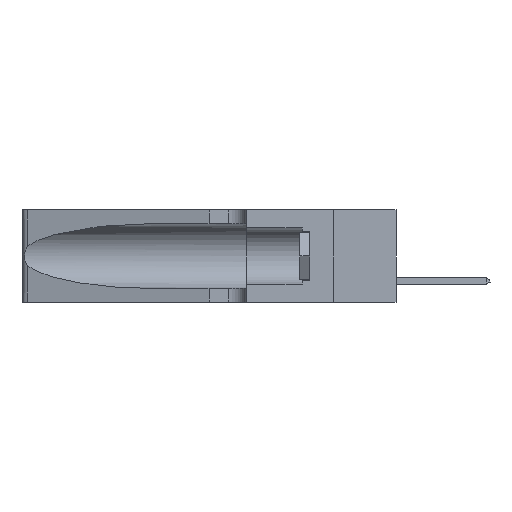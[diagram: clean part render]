
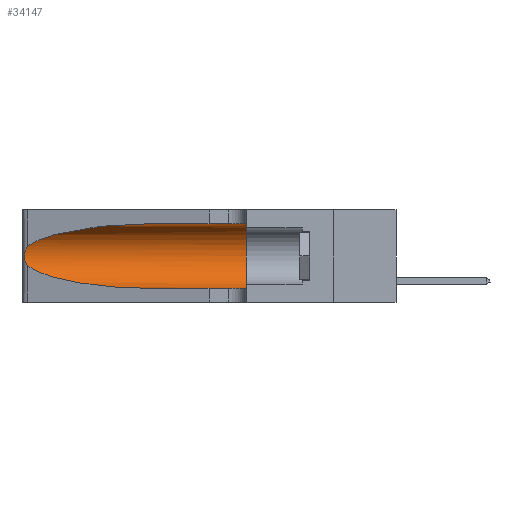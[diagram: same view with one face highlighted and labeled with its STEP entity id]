
A CAD part, left-side view. The second image highlights one B-rep face of the part: STEP entity #34147.
In plain terms, the highlighted cylindrical face has radius 3.308 mm (diameter 6.617 mm), a partial arc.
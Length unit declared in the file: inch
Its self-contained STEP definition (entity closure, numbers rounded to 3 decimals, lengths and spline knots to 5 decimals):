
#1822 = CARTESIAN_POINT ( 'NONE',  ( 0.26075, 1.23896, 0.19203 ) ) ;
#2509 = VERTEX_POINT ( 'NONE', #43721 ) ;
#2954 = CARTESIAN_POINT ( 'NONE',  ( 0.25487, 1.22718, 0.14631 ) ) ;
#3965 = EDGE_CURVE ( 'NONE', #22481, #14237, #27030, .T. ) ;
#4423 = DIRECTION ( 'NONE',  ( 0., -1., 0. ) ) ;
#4747 = DIRECTION ( 'NONE',  ( 0., 0., 1. ) ) ;
#7066 = CARTESIAN_POINT ( 'NONE',  ( 0.1305, 1.61858, 0.05475 ) ) ;
#9510 = CARTESIAN_POINT ( 'NONE',  ( 0.25854, 1.2359, 0.20912 ) ) ;
#10768 = CARTESIAN_POINT ( 'NONE',  ( 0.1305, 0.35, 0.05475 ) ) ;
#11154 = AXIS2_PLACEMENT_3D ( 'NONE', #19629, #4423, #23589 ) ;
#11292 = CARTESIAN_POINT ( 'NONE',  ( 0.2373, 1.15595, 0.28018 ) ) ;
#11744 = VECTOR ( 'NONE', #33843, 39.37008 ) ;
#12352 = CARTESIAN_POINT ( 'NONE',  ( 0.18966, 0.96281, 0.05475 ) ) ;
#12610 = CARTESIAN_POINT ( 'NONE',  ( 0.1305, 0.35, 0.31525 ) ) ;
#13565 = CYLINDRICAL_SURFACE ( 'NONE', #11154, 0.13025 ) ;
#13801 = CARTESIAN_POINT ( 'NONE',  ( 0.25787, 1.23484, 0.2124 ) ) ;
#14031 = EDGE_LOOP ( 'NONE', ( #42541, #44381, #28350, #35764, #25057, #31098 ) ) ;
#14237 = VERTEX_POINT ( 'NONE', #10768 ) ;
#14558 = CARTESIAN_POINT ( 'NONE',  ( 0.1305, 1.61858, 0.31525 ) ) ;
#16860 = CARTESIAN_POINT ( 'NONE',  ( 0.25789, 1.23486, 0.15765 ) ) ;
#16903 = AXIS2_PLACEMENT_3D ( 'NONE', #48190, #36298, #4747 ) ;
#16908 = EDGE_CURVE ( 'NONE', #50445, #22481, #19833, .T. ) ;
#17545 = VERTEX_POINT ( 'NONE', #22897 ) ;
#19164 = EDGE_CURVE ( 'NONE', #2509, #50445, #31392, .T. ) ;
#19212 =( BOUNDED_CURVE ( )  B_SPLINE_CURVE ( 3, ( #34308, #22917, #11292, #33979 ),
 .UNSPECIFIED., .F., .T. ) 
 B_SPLINE_CURVE_WITH_KNOTS ( ( 4, 4 ),
 ( 1.5708, 2.84003 ),
 .UNSPECIFIED. ) 
 CURVE ( )  GEOMETRIC_REPRESENTATION_ITEM ( )  RATIONAL_B_SPLINE_CURVE ( ( 1., 0.87, 0.87, 1. ) ) 
 REPRESENTATION_ITEM ( '' )  );
#19629 = CARTESIAN_POINT ( 'NONE',  ( 0.1305, 1.61858, 0.185 ) ) ;
#19833 =( BOUNDED_CURVE ( )  B_SPLINE_CURVE ( 3, ( #22563, #24682, #12352, #26880 ),
 .UNSPECIFIED., .F., .T. ) 
 B_SPLINE_CURVE_WITH_KNOTS ( ( 4, 4 ),
 ( 3.44316, 4.71239 ),
 .UNSPECIFIED. ) 
 CURVE ( )  GEOMETRIC_REPRESENTATION_ITEM ( )  RATIONAL_B_SPLINE_CURVE ( ( 1., 0.87, 0.87, 1. ) ) 
 REPRESENTATION_ITEM ( '' )  );
#20333 = VERTEX_POINT ( 'NONE', #12610 ) ;
#20903 = FACE_OUTER_BOUND ( 'NONE', #14031, .T. ) ;
#20957 = CARTESIAN_POINT ( 'NONE',  ( 0.25639, 1.23186, 0.15144 ) ) ;
#21315 = CARTESIAN_POINT ( 'NONE',  ( 0.26018, 1.23835, 0.19895 ) ) ;
#22481 = VERTEX_POINT ( 'NONE', #28026 ) ;
#22563 = CARTESIAN_POINT ( 'NONE',  ( 0.25487, 1.22718, 0.14631 ) ) ;
#22897 = CARTESIAN_POINT ( 'NONE',  ( 0.1305, 0.72297, 0.31525 ) ) ;
#22917 = CARTESIAN_POINT ( 'NONE',  ( 0.18966, 0.96281, 0.31525 ) ) ;
#23589 = DIRECTION ( 'NONE',  ( 0., 0., -1. ) ) ;
#24682 = CARTESIAN_POINT ( 'NONE',  ( 0.2373, 1.15595, 0.08982 ) ) ;
#25057 = ORIENTED_EDGE ( 'NONE', *, *, #42349, .F. ) ;
#26454 = LINE ( 'NONE', #14558, #49587 ) ;
#26880 = CARTESIAN_POINT ( 'NONE',  ( 0.1305, 0.72297, 0.05475 ) ) ;
#27030 = LINE ( 'NONE', #7066, #11744 ) ;
#28026 = CARTESIAN_POINT ( 'NONE',  ( 0.1305, 0.72297, 0.05475 ) ) ;
#28350 = ORIENTED_EDGE ( 'NONE', *, *, #16908, .T. ) ;
#29340 = EDGE_CURVE ( 'NONE', #17545, #2509, #19212, .T. ) ;
#29400 = EDGE_CURVE ( 'NONE', #17545, #20333, #26454, .T. ) ;
#31098 = ORIENTED_EDGE ( 'NONE', *, *, #29400, .F. ) ;
#31392 = B_SPLINE_CURVE_WITH_KNOTS ( 'NONE', 3,
 ( #39600, #32230, #40273, #13801, #9510, #21315, #1822, #41090, #42310, #36297, #16860, #20957, #45116, #38192 ),
 .UNSPECIFIED., .F., .F.,
 ( 4, 2, 2, 2, 2, 2, 4 ),
 ( 0., 0.00027, 0.00053, 0.00107, 0.0016, 0.00187, 0.00214 ),
 .UNSPECIFIED. ) ;
#32230 = CARTESIAN_POINT ( 'NONE',  ( 0.25555, 1.22994, 0.2215 ) ) ;
#33843 = DIRECTION ( 'NONE',  ( 0., -1., 0. ) ) ;
#33979 = CARTESIAN_POINT ( 'NONE',  ( 0.25487, 1.22718, 0.22369 ) ) ;
#34147 = ADVANCED_FACE ( 'NONE', ( #20903 ), #13565, .F. ) ;
#34308 = CARTESIAN_POINT ( 'NONE',  ( 0.1305, 0.72297, 0.31525 ) ) ;
#34813 = CIRCLE ( 'NONE', #16903, 0.13025 ) ;
#35764 = ORIENTED_EDGE ( 'NONE', *, *, #3965, .T. ) ;
#36297 = CARTESIAN_POINT ( 'NONE',  ( 0.25856, 1.23593, 0.16098 ) ) ;
#36298 = DIRECTION ( 'NONE',  ( 0., 1., 0. ) ) ;
#38192 = CARTESIAN_POINT ( 'NONE',  ( 0.25487, 1.22718, 0.14631 ) ) ;
#39600 = CARTESIAN_POINT ( 'NONE',  ( 0.25487, 1.22718, 0.22369 ) ) ;
#40273 = CARTESIAN_POINT ( 'NONE',  ( 0.25639, 1.23184, 0.21858 ) ) ;
#41090 = CARTESIAN_POINT ( 'NONE',  ( 0.26075, 1.23896, 0.178 ) ) ;
#42168 = DIRECTION ( 'NONE',  ( 0., -1., 0. ) ) ;
#42310 = CARTESIAN_POINT ( 'NONE',  ( 0.26017, 1.23833, 0.17102 ) ) ;
#42349 = EDGE_CURVE ( 'NONE', #20333, #14237, #34813, .T. ) ;
#42541 = ORIENTED_EDGE ( 'NONE', *, *, #29340, .T. ) ;
#43721 = CARTESIAN_POINT ( 'NONE',  ( 0.25487, 1.22718, 0.22369 ) ) ;
#44381 = ORIENTED_EDGE ( 'NONE', *, *, #19164, .T. ) ;
#45116 = CARTESIAN_POINT ( 'NONE',  ( 0.25555, 1.22993, 0.14849 ) ) ;
#48190 = CARTESIAN_POINT ( 'NONE',  ( 0.1305, 0.35, 0.185 ) ) ;
#49587 = VECTOR ( 'NONE', #42168, 39.37008 ) ;
#50445 = VERTEX_POINT ( 'NONE', #2954 ) ;
